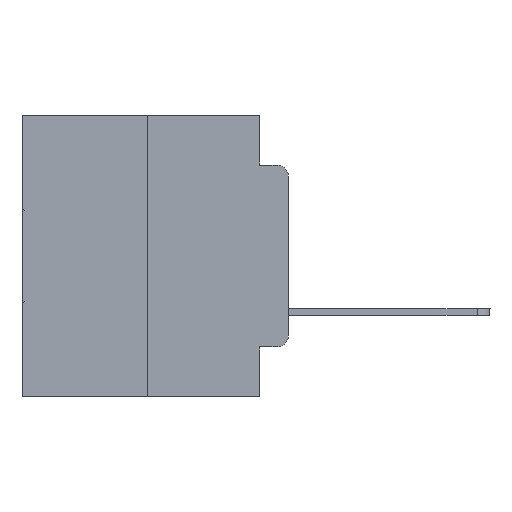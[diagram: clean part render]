
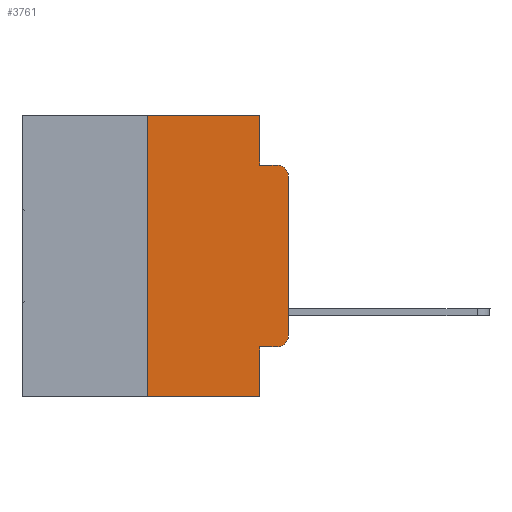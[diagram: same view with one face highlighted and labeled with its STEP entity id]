
A CAD part, left-side view. The second image highlights one B-rep face of the part: STEP entity #3761.
In plain terms, the highlighted planar face has unit normal (-1, 0, 0).
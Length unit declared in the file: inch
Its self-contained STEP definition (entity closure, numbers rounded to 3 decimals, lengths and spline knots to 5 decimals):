
#358 = LINE ( 'NONE', #17629, #24455 ) ;
#404 = LINE ( 'NONE', #26161, #21948 ) ;
#709 = EDGE_CURVE ( 'NONE', #21127, #23078, #11443, .T. ) ;
#1775 = ORIENTED_EDGE ( 'NONE', *, *, #11002, .T. ) ;
#2189 = EDGE_CURVE ( 'NONE', #13727, #23164, #11727, .T. ) ;
#2484 = LINE ( 'NONE', #10589, #7864 ) ;
#3463 = CARTESIAN_POINT ( 'NONE',  ( 0., 0.473, 0. ) ) ;
#3761 = ADVANCED_FACE ( 'NONE', ( #26349 ), #12526, .F. ) ;
#3990 = CARTESIAN_POINT ( 'NONE',  ( 0., 0.25, -0.5 ) ) ;
#4272 = CARTESIAN_POINT ( 'NONE',  ( 0., 0.051, -0.4115 ) ) ;
#4871 = ORIENTED_EDGE ( 'NONE', *, *, #24918, .F. ) ;
#5240 = EDGE_CURVE ( 'NONE', #28366, #6531, #404, .T. ) ;
#5437 = CARTESIAN_POINT ( 'NONE',  ( 0., 0.051, 0. ) ) ;
#5514 = DIRECTION ( 'NONE',  ( -1., 0., 0. ) ) ;
#5812 = CARTESIAN_POINT ( 'NONE',  ( 0., 0.051, 0. ) ) ;
#6531 = VERTEX_POINT ( 'NONE', #26054 ) ;
#6968 = CARTESIAN_POINT ( 'NONE',  ( 0., 0., 0. ) ) ;
#7018 = DIRECTION ( 'NONE',  ( 0., -1., 0. ) ) ;
#7307 = ORIENTED_EDGE ( 'NONE', *, *, #24646, .F. ) ;
#7639 = DIRECTION ( 'NONE',  ( 0., 0., 1. ) ) ;
#7864 = VECTOR ( 'NONE', #19868, 39.37008 ) ;
#8916 = AXIS2_PLACEMENT_3D ( 'NONE', #23707, #5514, #12447 ) ;
#9306 = VECTOR ( 'NONE', #26141, 39.37008 ) ;
#9348 = VERTEX_POINT ( 'NONE', #11801 ) ;
#9380 = VECTOR ( 'NONE', #12252, 39.37008 ) ;
#9669 = LINE ( 'NONE', #6968, #17299 ) ;
#10254 = ORIENTED_EDGE ( 'NONE', *, *, #2189, .T. ) ;
#10459 = VERTEX_POINT ( 'NONE', #27765 ) ;
#10574 = LINE ( 'NONE', #26329, #9380 ) ;
#10589 = CARTESIAN_POINT ( 'NONE',  ( 0., 0.051, -0.0885 ) ) ;
#11002 = EDGE_CURVE ( 'NONE', #21127, #13727, #358, .T. ) ;
#11034 = DIRECTION ( 'NONE',  ( 0., 0., -1. ) ) ;
#11055 = EDGE_CURVE ( 'NONE', #23164, #9348, #9669, .T. ) ;
#11443 = LINE ( 'NONE', #5812, #29082 ) ;
#11727 = CIRCLE ( 'NONE', #8916, 0.02 ) ;
#11801 = CARTESIAN_POINT ( 'NONE',  ( 0., 0., -0.1085 ) ) ;
#12252 = DIRECTION ( 'NONE',  ( 0., -1., 0. ) ) ;
#12447 = DIRECTION ( 'NONE',  ( 0., 0., -1. ) ) ;
#12526 = PLANE ( 'NONE',  #19952 ) ;
#13051 = AXIS2_PLACEMENT_3D ( 'NONE', #19426, #21497, #23713 ) ;
#13727 = VERTEX_POINT ( 'NONE', #16228 ) ;
#14496 = CARTESIAN_POINT ( 'NONE',  ( 0., 0.051, -0.5 ) ) ;
#16228 = CARTESIAN_POINT ( 'NONE',  ( 0., 0.02, -0.4115 ) ) ;
#17078 = VERTEX_POINT ( 'NONE', #29770 ) ;
#17299 = VECTOR ( 'NONE', #27712, 39.37008 ) ;
#17629 = CARTESIAN_POINT ( 'NONE',  ( 0., 0.051, -0.4115 ) ) ;
#18127 = EDGE_CURVE ( 'NONE', #6531, #17078, #10574, .T. ) ;
#18539 = CARTESIAN_POINT ( 'NONE',  ( 0., 0.473, -0.5 ) ) ;
#19095 = ORIENTED_EDGE ( 'NONE', *, *, #27912, .T. ) ;
#19426 = CARTESIAN_POINT ( 'NONE',  ( 0., 0.02, -0.1085 ) ) ;
#19717 = CIRCLE ( 'NONE', #13051, 0.02 ) ;
#19868 = DIRECTION ( 'NONE',  ( 0., -1., 0. ) ) ;
#19952 = AXIS2_PLACEMENT_3D ( 'NONE', #3463, #28501, #21759 ) ;
#20727 = ORIENTED_EDGE ( 'NONE', *, *, #11055, .T. ) ;
#20819 = ORIENTED_EDGE ( 'NONE', *, *, #26740, .T. ) ;
#21127 = VERTEX_POINT ( 'NONE', #4272 ) ;
#21217 = CARTESIAN_POINT ( 'NONE',  ( 0., 0., -0.3915 ) ) ;
#21497 = DIRECTION ( 'NONE',  ( -1., 0., 0. ) ) ;
#21759 = DIRECTION ( 'NONE',  ( 0., 0., -1. ) ) ;
#21948 = VECTOR ( 'NONE', #7639, 39.37008 ) ;
#22930 = CARTESIAN_POINT ( 'NONE',  ( 0., 0.051, -0.0885 ) ) ;
#22969 = ORIENTED_EDGE ( 'NONE', *, *, #18127, .F. ) ;
#23078 = VERTEX_POINT ( 'NONE', #14496 ) ;
#23164 = VERTEX_POINT ( 'NONE', #21217 ) ;
#23605 = LINE ( 'NONE', #18539, #26514 ) ;
#23707 = CARTESIAN_POINT ( 'NONE',  ( 0., 0.02, -0.3915 ) ) ;
#23713 = DIRECTION ( 'NONE',  ( 0., 0., -1. ) ) ;
#24455 = VECTOR ( 'NONE', #29234, 39.37008 ) ;
#24646 = EDGE_CURVE ( 'NONE', #29213, #10459, #2484, .T. ) ;
#24918 = EDGE_CURVE ( 'NONE', #17078, #29213, #27681, .T. ) ;
#26054 = CARTESIAN_POINT ( 'NONE',  ( 0., 0.25, 0. ) ) ;
#26141 = DIRECTION ( 'NONE',  ( 0., 0., -1. ) ) ;
#26161 = CARTESIAN_POINT ( 'NONE',  ( 0., 0.25, 0. ) ) ;
#26329 = CARTESIAN_POINT ( 'NONE',  ( 0., 0.473, 0. ) ) ;
#26349 = FACE_OUTER_BOUND ( 'NONE', #27020, .T. ) ;
#26514 = VECTOR ( 'NONE', #7018, 39.37008 ) ;
#26740 = EDGE_CURVE ( 'NONE', #28366, #23078, #23605, .T. ) ;
#26784 = ORIENTED_EDGE ( 'NONE', *, *, #709, .F. ) ;
#26948 = ORIENTED_EDGE ( 'NONE', *, *, #5240, .F. ) ;
#27020 = EDGE_LOOP ( 'NONE', ( #20727, #19095, #7307, #4871, #22969, #26948, #20819, #26784, #1775, #10254 ) ) ;
#27681 = LINE ( 'NONE', #5437, #9306 ) ;
#27712 = DIRECTION ( 'NONE',  ( 0., 0., 1. ) ) ;
#27765 = CARTESIAN_POINT ( 'NONE',  ( 0., 0.02, -0.0885 ) ) ;
#27912 = EDGE_CURVE ( 'NONE', #9348, #10459, #19717, .T. ) ;
#28366 = VERTEX_POINT ( 'NONE', #3990 ) ;
#28501 = DIRECTION ( 'NONE',  ( 1., 0., 0. ) ) ;
#29082 = VECTOR ( 'NONE', #11034, 39.37008 ) ;
#29213 = VERTEX_POINT ( 'NONE', #22930 ) ;
#29234 = DIRECTION ( 'NONE',  ( 0., -1., 0. ) ) ;
#29770 = CARTESIAN_POINT ( 'NONE',  ( 0., 0.051, 0. ) ) ;
